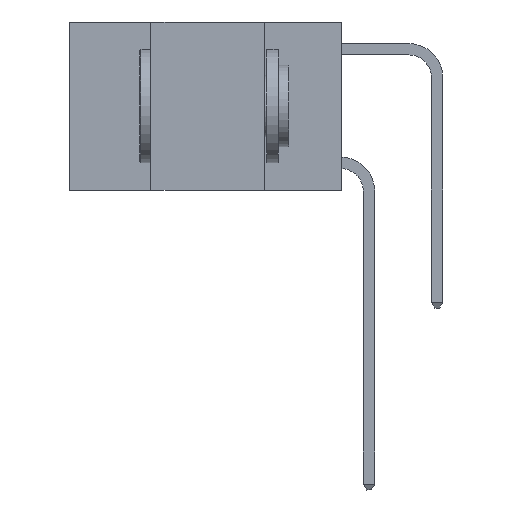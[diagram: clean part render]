
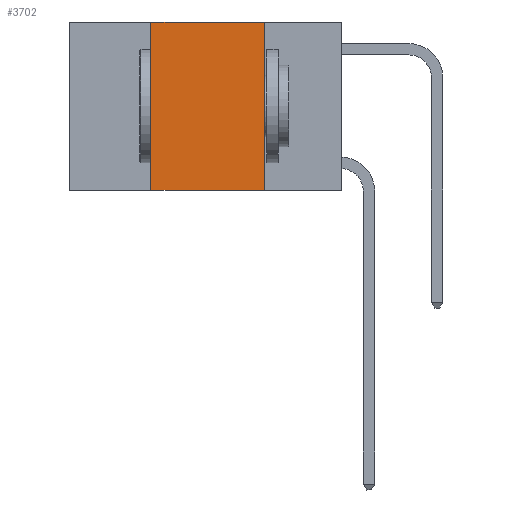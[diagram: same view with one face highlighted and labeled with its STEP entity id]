
A CAD part, left-side view. The second image highlights one B-rep face of the part: STEP entity #3702.
In plain terms, the highlighted planar face has unit normal (-1, 0, 0).
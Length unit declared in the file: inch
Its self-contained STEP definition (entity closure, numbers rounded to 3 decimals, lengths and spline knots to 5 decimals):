
#130 = LINE ( 'NONE', #3951, #1659 ) ;
#209 = FACE_OUTER_BOUND ( 'NONE', #10705, .T. ) ;
#214 = LINE ( 'NONE', #4038, #343 ) ;
#329 = DIRECTION ( 'NONE',  ( 0., 0., -1. ) ) ;
#343 = VECTOR ( 'NONE', #7810, 39.37008 ) ;
#1401 = CARTESIAN_POINT ( 'NONE',  ( 0., 0.17, 0. ) ) ;
#1419 = EDGE_CURVE ( 'NONE', #1530, #3747, #214, .T. ) ;
#1530 = VERTEX_POINT ( 'NONE', #8978 ) ;
#1547 = CARTESIAN_POINT ( 'NONE',  ( 0., 0.6, 0. ) ) ;
#1641 = DIRECTION ( 'NONE',  ( 0., 0., 1. ) ) ;
#1659 = VECTOR ( 'NONE', #6791, 39.37008 ) ;
#2801 = ORIENTED_EDGE ( 'NONE', *, *, #3839, .F. ) ;
#2872 = VERTEX_POINT ( 'NONE', #1401 ) ;
#2925 = VECTOR ( 'NONE', #1641, 39.37008 ) ;
#3216 = PLANE ( 'NONE',  #5545 ) ;
#3236 = ORIENTED_EDGE ( 'NONE', *, *, #1419, .T. ) ;
#3702 = ADVANCED_FACE ( 'NONE', ( #209 ), #3216, .F. ) ;
#3747 = VERTEX_POINT ( 'NONE', #4033 ) ;
#3839 = EDGE_CURVE ( 'NONE', #1530, #4312, #8972, .T. ) ;
#3951 = CARTESIAN_POINT ( 'NONE',  ( 0., 0.17, 0. ) ) ;
#4033 = CARTESIAN_POINT ( 'NONE',  ( 0., 0.17, -0.37 ) ) ;
#4038 = CARTESIAN_POINT ( 'NONE',  ( 0., 0.6, -0.37 ) ) ;
#4077 = ORIENTED_EDGE ( 'NONE', *, *, #10599, .F. ) ;
#4312 = VERTEX_POINT ( 'NONE', #8263 ) ;
#4412 = DIRECTION ( 'NONE',  ( 0., -1., 0. ) ) ;
#5368 = VECTOR ( 'NONE', #4412, 39.37008 ) ;
#5545 = AXIS2_PLACEMENT_3D ( 'NONE', #8791, #8859, #329 ) ;
#6065 = EDGE_CURVE ( 'NONE', #2872, #3747, #130, .T. ) ;
#6791 = DIRECTION ( 'NONE',  ( 0., 0., -1. ) ) ;
#7810 = DIRECTION ( 'NONE',  ( 0., -1., 0. ) ) ;
#8263 = CARTESIAN_POINT ( 'NONE',  ( 0., 0.42, 0. ) ) ;
#8791 = CARTESIAN_POINT ( 'NONE',  ( 0., 0.6, 0. ) ) ;
#8859 = DIRECTION ( 'NONE',  ( 1., 0., 0. ) ) ;
#8972 = LINE ( 'NONE', #9102, #2925 ) ;
#8978 = CARTESIAN_POINT ( 'NONE',  ( 0., 0.42, -0.37 ) ) ;
#9102 = CARTESIAN_POINT ( 'NONE',  ( 0., 0.42, 0. ) ) ;
#10275 = ORIENTED_EDGE ( 'NONE', *, *, #6065, .F. ) ;
#10599 = EDGE_CURVE ( 'NONE', #4312, #2872, #11265, .T. ) ;
#10705 = EDGE_LOOP ( 'NONE', ( #10275, #4077, #2801, #3236 ) ) ;
#11265 = LINE ( 'NONE', #1547, #5368 ) ;
